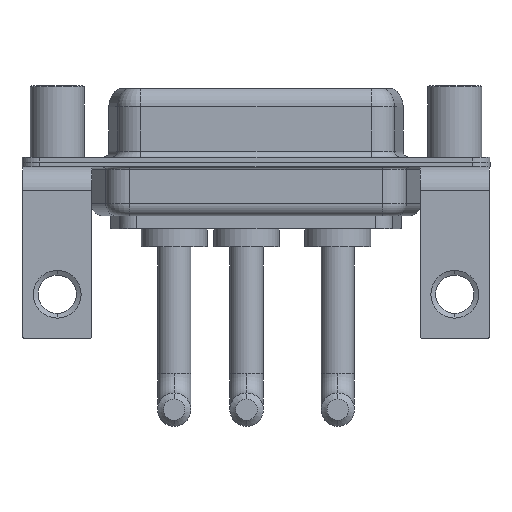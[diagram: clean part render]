
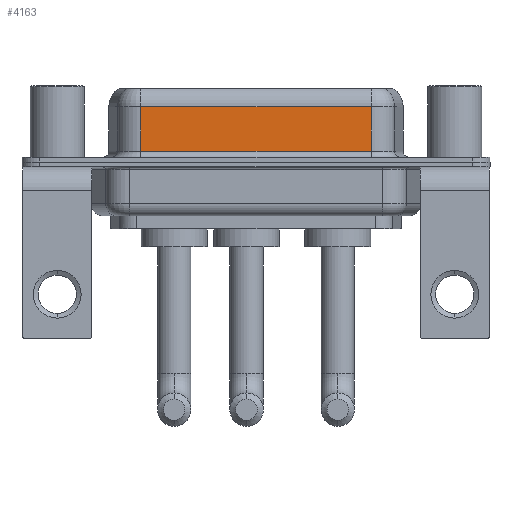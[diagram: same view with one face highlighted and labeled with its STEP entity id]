
A CAD part, front view. The second image highlights one B-rep face of the part: STEP entity #4163.
In plain terms, the highlighted planar face has unit normal (0, -1, 0).
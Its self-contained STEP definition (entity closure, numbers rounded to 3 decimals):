
#142 = DIRECTION ( 'NONE',  ( 0., 0., -1. ) ) ;
#323 = CARTESIAN_POINT ( 'NONE',  ( 26.287, -3.95, 6.4 ) ) ;
#565 = DIRECTION ( 'NONE',  ( 0., 0., -1. ) ) ;
#2945 = FACE_OUTER_BOUND ( 'NONE', #5121, .T. ) ;
#3023 = CARTESIAN_POINT ( 'NONE',  ( 26.287, -3.95, 6.4 ) ) ;
#3298 = VECTOR ( 'NONE', #14692, 1000. ) ;
#3489 = CARTESIAN_POINT ( 'NONE',  ( 26.287, -3.95, 0.9 ) ) ;
#3548 = ORIENTED_EDGE ( 'NONE', *, *, #5693, .T. ) ;
#4163 = ADVANCED_FACE ( 'NONE', ( #2945 ), #6715, .F. ) ;
#4632 = CARTESIAN_POINT ( 'NONE',  ( 26.287, -3.95, 4.65 ) ) ;
#4737 = ORIENTED_EDGE ( 'NONE', *, *, #15189, .F. ) ;
#5121 = EDGE_LOOP ( 'NONE', ( #4737, #6338, #3548, #10999 ) ) ;
#5124 = VERTEX_POINT ( 'NONE', #6297 ) ;
#5537 = DIRECTION ( 'NONE',  ( 0., 0., 1. ) ) ;
#5693 = EDGE_CURVE ( 'NONE', #13927, #5124, #11539, .T. ) ;
#5917 = DIRECTION ( 'NONE',  ( 1., 0., 0. ) ) ;
#6043 = CARTESIAN_POINT ( 'NONE',  ( 7.013, -3.95, 4.65 ) ) ;
#6297 = CARTESIAN_POINT ( 'NONE',  ( 7.013, -3.95, 0.9 ) ) ;
#6338 = ORIENTED_EDGE ( 'NONE', *, *, #8644, .T. ) ;
#6715 = PLANE ( 'NONE',  #12702 ) ;
#8243 = VECTOR ( 'NONE', #142, 1000. ) ;
#8306 = EDGE_CURVE ( 'NONE', #5124, #13567, #10867, .T. ) ;
#8644 = EDGE_CURVE ( 'NONE', #11941, #13927, #14775, .T. ) ;
#8729 = VECTOR ( 'NONE', #565, 1000. ) ;
#9648 = DIRECTION ( 'NONE',  ( 0., 1., 0. ) ) ;
#10023 = CARTESIAN_POINT ( 'NONE',  ( 26.287, -3.95, 0.9 ) ) ;
#10691 = VECTOR ( 'NONE', #5917, 1000. ) ;
#10867 = LINE ( 'NONE', #3489, #10691 ) ;
#10999 = ORIENTED_EDGE ( 'NONE', *, *, #8306, .T. ) ;
#11539 = LINE ( 'NONE', #13915, #8243 ) ;
#11555 = LINE ( 'NONE', #323, #8729 ) ;
#11941 = VERTEX_POINT ( 'NONE', #15758 ) ;
#12702 = AXIS2_PLACEMENT_3D ( 'NONE', #3023, #9648, #5537 ) ;
#13567 = VERTEX_POINT ( 'NONE', #10023 ) ;
#13915 = CARTESIAN_POINT ( 'NONE',  ( 7.013, -3.95, 6.4 ) ) ;
#13927 = VERTEX_POINT ( 'NONE', #6043 ) ;
#14692 = DIRECTION ( 'NONE',  ( -1., 0., 0. ) ) ;
#14775 = LINE ( 'NONE', #4632, #3298 ) ;
#15189 = EDGE_CURVE ( 'NONE', #11941, #13567, #11555, .T. ) ;
#15758 = CARTESIAN_POINT ( 'NONE',  ( 26.287, -3.95, 4.65 ) ) ;
